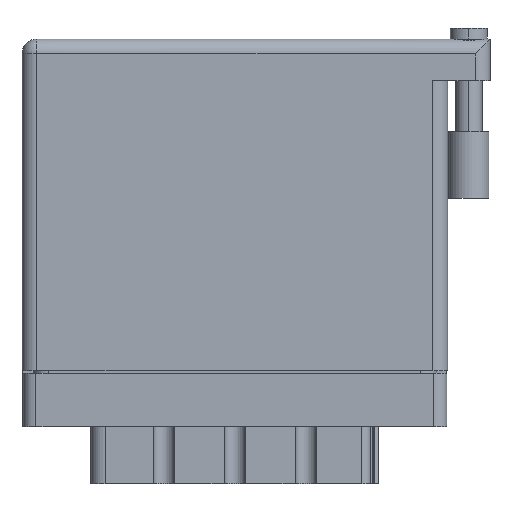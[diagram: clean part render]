
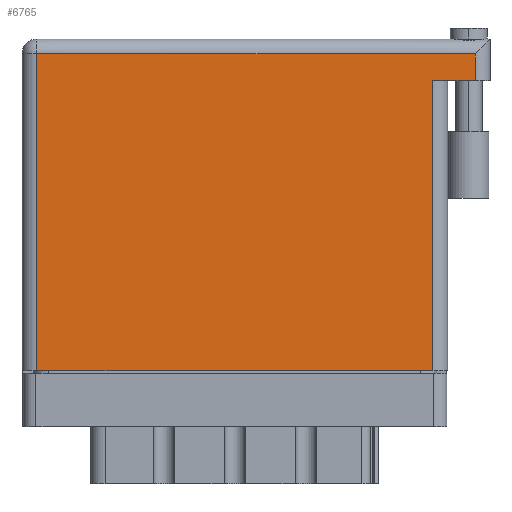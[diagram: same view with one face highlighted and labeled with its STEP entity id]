
A CAD part, front view. The second image highlights one B-rep face of the part: STEP entity #6765.
In plain terms, the highlighted face is planar.
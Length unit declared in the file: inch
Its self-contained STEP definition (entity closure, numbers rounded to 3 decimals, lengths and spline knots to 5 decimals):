
#446 = VECTOR ( 'NONE', #15106, 39.37008 ) ;
#1187 = DIRECTION ( 'NONE',  ( 0., 1., 0. ) ) ;
#2559 = CARTESIAN_POINT ( 'NONE',  ( 2.208, 1.369, 0. ) ) ;
#3099 = VERTEX_POINT ( 'NONE', #31847 ) ;
#4715 = EDGE_CURVE ( 'NONE', #26087, #10973, #9492, .T. ) ;
#5209 = VERTEX_POINT ( 'NONE', #22993 ) ;
#5921 = ORIENTED_EDGE ( 'NONE', *, *, #32857, .T. ) ;
#6068 = CARTESIAN_POINT ( 'NONE',  ( 0., 1.566, 0. ) ) ;
#6181 = CARTESIAN_POINT ( 'NONE',  ( 0., 1.496, 0. ) ) ;
#6765 = ADVANCED_FACE ( 'NONE', ( #40914 ), #34236, .F. ) ;
#7452 = ORIENTED_EDGE ( 'NONE', *, *, #21838, .T. ) ;
#7761 = ORIENTED_EDGE ( 'NONE', *, *, #4715, .T. ) ;
#7930 = ORIENTED_EDGE ( 'NONE', *, *, #40924, .F. ) ;
#8675 = CARTESIAN_POINT ( 'NONE',  ( 2.138, 1.566, 0. ) ) ;
#9492 = LINE ( 'NONE', #25248, #23873 ) ;
#10973 = VERTEX_POINT ( 'NONE', #23728 ) ;
#12586 = LINE ( 'NONE', #37927, #36797 ) ;
#13402 = EDGE_CURVE ( 'NONE', #5209, #26087, #12586, .T. ) ;
#13744 = VECTOR ( 'NONE', #38546, 39.37008 ) ;
#15106 = DIRECTION ( 'NONE',  ( -1., 0., 0. ) ) ;
#15555 = DIRECTION ( 'NONE',  ( 1., 0., 0. ) ) ;
#15596 = DIRECTION ( 'NONE',  ( -1., 0., 0. ) ) ;
#15990 = VECTOR ( 'NONE', #30723, 39.37008 ) ;
#16321 = CARTESIAN_POINT ( 'NONE',  ( 0.07, 0., 0. ) ) ;
#17281 = ORIENTED_EDGE ( 'NONE', *, *, #30424, .T. ) ;
#17937 = VECTOR ( 'NONE', #1187, 39.37008 ) ;
#18144 = VERTEX_POINT ( 'NONE', #21798 ) ;
#19733 = ORIENTED_EDGE ( 'NONE', *, *, #13402, .T. ) ;
#21175 = LINE ( 'NONE', #2559, #446 ) ;
#21798 = CARTESIAN_POINT ( 'NONE',  ( 2.138, 1.496, 0. ) ) ;
#21838 = EDGE_CURVE ( 'NONE', #10973, #22595, #35765, .T. ) ;
#22595 = VERTEX_POINT ( 'NONE', #24101 ) ;
#22993 = CARTESIAN_POINT ( 'NONE',  ( 0.07, 1.496, 0. ) ) ;
#23312 = CARTESIAN_POINT ( 'NONE',  ( 1.938, 1.369, 0. ) ) ;
#23728 = CARTESIAN_POINT ( 'NONE',  ( 1.938, 0., 0. ) ) ;
#23873 = VECTOR ( 'NONE', #15555, 39.37008 ) ;
#24101 = CARTESIAN_POINT ( 'NONE',  ( 1.938, 1.369, 0. ) ) ;
#24436 = LINE ( 'NONE', #8675, #15990 ) ;
#25248 = CARTESIAN_POINT ( 'NONE',  ( 0., 0., 0. ) ) ;
#26087 = VERTEX_POINT ( 'NONE', #16321 ) ;
#27126 = LINE ( 'NONE', #6181, #13744 ) ;
#27441 = EDGE_LOOP ( 'NONE', ( #7761, #7452, #7930, #5921, #17281, #19733 ) ) ;
#30424 = EDGE_CURVE ( 'NONE', #18144, #5209, #27126, .T. ) ;
#30723 = DIRECTION ( 'NONE',  ( 0., 1., 0. ) ) ;
#31692 = DIRECTION ( 'NONE',  ( 0., -1., 0. ) ) ;
#31847 = CARTESIAN_POINT ( 'NONE',  ( 2.138, 1.369, 0. ) ) ;
#32505 = AXIS2_PLACEMENT_3D ( 'NONE', #6068, #37264, #15596 ) ;
#32857 = EDGE_CURVE ( 'NONE', #3099, #18144, #24436, .T. ) ;
#34236 = PLANE ( 'NONE',  #32505 ) ;
#35765 = LINE ( 'NONE', #23312, #17937 ) ;
#36797 = VECTOR ( 'NONE', #31692, 39.37008 ) ;
#37264 = DIRECTION ( 'NONE',  ( 0., 0., -1. ) ) ;
#37927 = CARTESIAN_POINT ( 'NONE',  ( 0.07, 0., 0. ) ) ;
#38546 = DIRECTION ( 'NONE',  ( -1., 0., 0. ) ) ;
#40914 = FACE_OUTER_BOUND ( 'NONE', #27441, .T. ) ;
#40924 = EDGE_CURVE ( 'NONE', #3099, #22595, #21175, .T. ) ;
